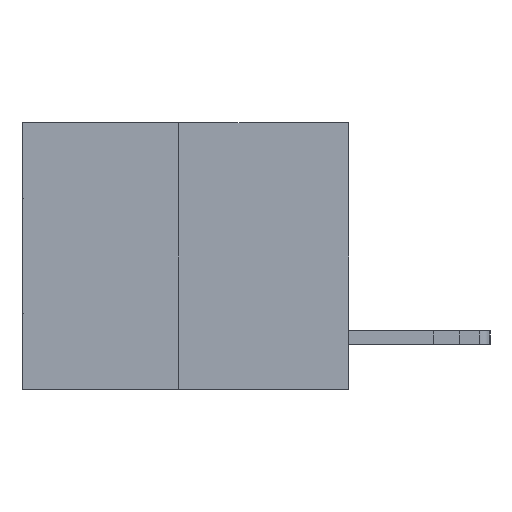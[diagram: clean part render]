
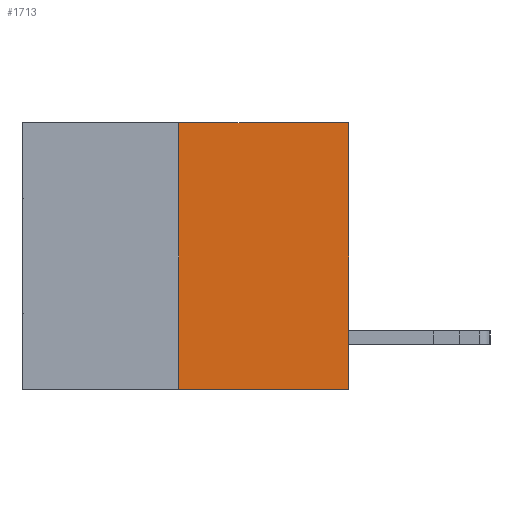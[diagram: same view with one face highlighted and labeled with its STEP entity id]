
A CAD part, left-side view. The second image highlights one B-rep face of the part: STEP entity #1713.
In plain terms, the highlighted planar face has unit normal (-1, 0, 0).
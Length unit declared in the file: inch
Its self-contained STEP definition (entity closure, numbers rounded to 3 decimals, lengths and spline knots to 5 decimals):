
#4 = EDGE_CURVE ( 'NONE', #20082, #24344, #26521, .T. ) ;
#1713 = ADVANCED_FACE ( 'NONE', ( #11086 ), #19205, .F. ) ;
#4053 = CARTESIAN_POINT ( 'NONE',  ( 0., 0.312, 0. ) ) ;
#4724 = VERTEX_POINT ( 'NONE', #6620 ) ;
#4965 = ORIENTED_EDGE ( 'NONE', *, *, #4, .F. ) ;
#6620 = CARTESIAN_POINT ( 'NONE',  ( 0., 0., -0.49 ) ) ;
#8588 = VECTOR ( 'NONE', #12525, 39.37008 ) ;
#9728 = AXIS2_PLACEMENT_3D ( 'NONE', #9822, #14306, #12141 ) ;
#9822 = CARTESIAN_POINT ( 'NONE',  ( 0., 0.6, 0. ) ) ;
#11086 = FACE_OUTER_BOUND ( 'NONE', #20985, .T. ) ;
#12141 = DIRECTION ( 'NONE',  ( 0., 0., -1. ) ) ;
#12525 = DIRECTION ( 'NONE',  ( 0., 0., 1. ) ) ;
#13259 = CARTESIAN_POINT ( 'NONE',  ( 0., 0.312, -0.49 ) ) ;
#13766 = EDGE_CURVE ( 'NONE', #4724, #24344, #30065, .T. ) ;
#13796 = VECTOR ( 'NONE', #21690, 39.37008 ) ;
#14306 = DIRECTION ( 'NONE',  ( 1., 0., 0. ) ) ;
#15453 = LINE ( 'NONE', #18460, #23451 ) ;
#16440 = DIRECTION ( 'NONE',  ( 0., 0., 1. ) ) ;
#17161 = CARTESIAN_POINT ( 'NONE',  ( 0., 0.6, -0.49 ) ) ;
#18460 = CARTESIAN_POINT ( 'NONE',  ( 0., 0.312, -0.49 ) ) ;
#18965 = ORIENTED_EDGE ( 'NONE', *, *, #19562, .F. ) ;
#19205 = PLANE ( 'NONE',  #9728 ) ;
#19562 = EDGE_CURVE ( 'NONE', #25625, #20082, #15453, .T. ) ;
#19871 = ORIENTED_EDGE ( 'NONE', *, *, #13766, .T. ) ;
#20082 = VERTEX_POINT ( 'NONE', #4053 ) ;
#20985 = EDGE_LOOP ( 'NONE', ( #18965, #29557, #19871, #4965 ) ) ;
#21690 = DIRECTION ( 'NONE',  ( 0., -1., 0. ) ) ;
#23451 = VECTOR ( 'NONE', #16440, 39.37008 ) ;
#24344 = VERTEX_POINT ( 'NONE', #25424 ) ;
#24383 = DIRECTION ( 'NONE',  ( 0., -1., 0. ) ) ;
#24744 = LINE ( 'NONE', #17161, #25091 ) ;
#25091 = VECTOR ( 'NONE', #24383, 39.37008 ) ;
#25424 = CARTESIAN_POINT ( 'NONE',  ( 0., 0., 0. ) ) ;
#25625 = VERTEX_POINT ( 'NONE', #13259 ) ;
#26478 = CARTESIAN_POINT ( 'NONE',  ( 0., 0., 0. ) ) ;
#26521 = LINE ( 'NONE', #28989, #13796 ) ;
#27003 = EDGE_CURVE ( 'NONE', #25625, #4724, #24744, .T. ) ;
#28989 = CARTESIAN_POINT ( 'NONE',  ( 0., 0.6, 0. ) ) ;
#29557 = ORIENTED_EDGE ( 'NONE', *, *, #27003, .T. ) ;
#30065 = LINE ( 'NONE', #26478, #8588 ) ;
